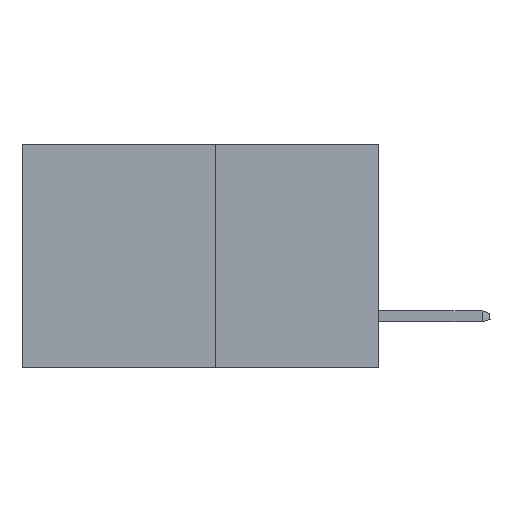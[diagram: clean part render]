
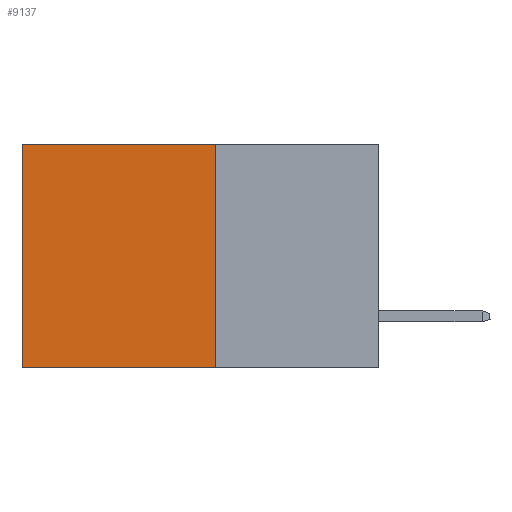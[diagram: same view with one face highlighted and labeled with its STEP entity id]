
A CAD part, left-side view. The second image highlights one B-rep face of the part: STEP entity #9137.
In plain terms, the highlighted planar face has unit normal (-1, 0, 0).
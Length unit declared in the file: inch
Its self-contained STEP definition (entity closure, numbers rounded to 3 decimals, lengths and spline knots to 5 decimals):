
#996 = DIRECTION ( 'NONE',  ( 0., 0., -1. ) ) ;
#1172 = CARTESIAN_POINT ( 'NONE',  ( 0.277, 0.27, -0.37 ) ) ;
#1183 = ORIENTED_EDGE ( 'NONE', *, *, #4506, .T. ) ;
#3226 = EDGE_CURVE ( 'NONE', #20412, #6488, #7400, .T. ) ;
#3804 = CARTESIAN_POINT ( 'NONE',  ( 0.277, 0.27, 0. ) ) ;
#4283 = VECTOR ( 'NONE', #14275, 39.37008 ) ;
#4506 = EDGE_CURVE ( 'NONE', #14061, #9595, #20210, .T. ) ;
#5913 = FACE_OUTER_BOUND ( 'NONE', #16785, .T. ) ;
#6488 = VERTEX_POINT ( 'NONE', #11103 ) ;
#7034 = EDGE_CURVE ( 'NONE', #14061, #20412, #12357, .T. ) ;
#7226 = PLANE ( 'NONE',  #18411 ) ;
#7297 = DIRECTION ( 'NONE',  ( 0., 0., -1. ) ) ;
#7400 = LINE ( 'NONE', #13419, #15525 ) ;
#7565 = CARTESIAN_POINT ( 'NONE',  ( 0.277, 0.27, 0. ) ) ;
#7945 = DIRECTION ( 'NONE',  ( 0., 1., 0. ) ) ;
#8277 = ORIENTED_EDGE ( 'NONE', *, *, #3226, .F. ) ;
#9106 = LINE ( 'NONE', #12685, #4283 ) ;
#9137 = ADVANCED_FACE ( 'NONE', ( #5913 ), #7226, .F. ) ;
#9595 = VERTEX_POINT ( 'NONE', #10095 ) ;
#10095 = CARTESIAN_POINT ( 'NONE',  ( 0.277, 0.59, 0. ) ) ;
#10516 = EDGE_CURVE ( 'NONE', #9595, #6488, #9106, .T. ) ;
#11103 = CARTESIAN_POINT ( 'NONE',  ( 0.277, 0.59, -0.37 ) ) ;
#11676 = VECTOR ( 'NONE', #7945, 39.37008 ) ;
#12357 = LINE ( 'NONE', #1172, #20843 ) ;
#12685 = CARTESIAN_POINT ( 'NONE',  ( 0.277, 0.59, -0.37 ) ) ;
#13245 = DIRECTION ( 'NONE',  ( 0., 1., 0. ) ) ;
#13419 = CARTESIAN_POINT ( 'NONE',  ( 0.277, 0.27, -0.37 ) ) ;
#14061 = VERTEX_POINT ( 'NONE', #3804 ) ;
#14275 = DIRECTION ( 'NONE',  ( 0., 0., -1. ) ) ;
#15378 = CARTESIAN_POINT ( 'NONE',  ( 0.277, 0.27, -0.37 ) ) ;
#15525 = VECTOR ( 'NONE', #13245, 39.37008 ) ;
#16785 = EDGE_LOOP ( 'NONE', ( #20158, #8277, #16947, #1183 ) ) ;
#16947 = ORIENTED_EDGE ( 'NONE', *, *, #7034, .F. ) ;
#17040 = DIRECTION ( 'NONE',  ( 1., 0., 0. ) ) ;
#18411 = AXIS2_PLACEMENT_3D ( 'NONE', #15378, #17040, #7297 ) ;
#20158 = ORIENTED_EDGE ( 'NONE', *, *, #10516, .T. ) ;
#20210 = LINE ( 'NONE', #7565, #11676 ) ;
#20412 = VERTEX_POINT ( 'NONE', #20542 ) ;
#20542 = CARTESIAN_POINT ( 'NONE',  ( 0.277, 0.27, -0.37 ) ) ;
#20843 = VECTOR ( 'NONE', #996, 39.37008 ) ;
